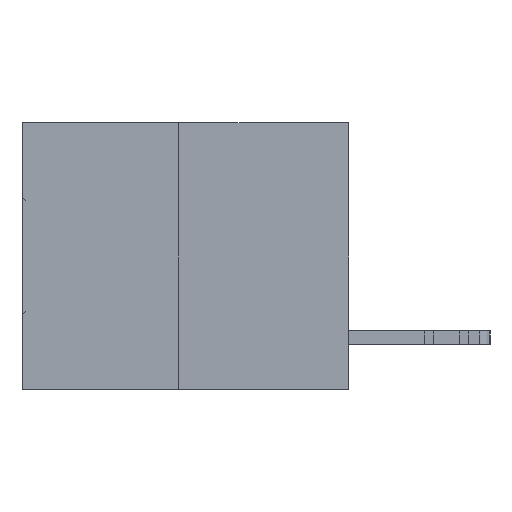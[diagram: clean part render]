
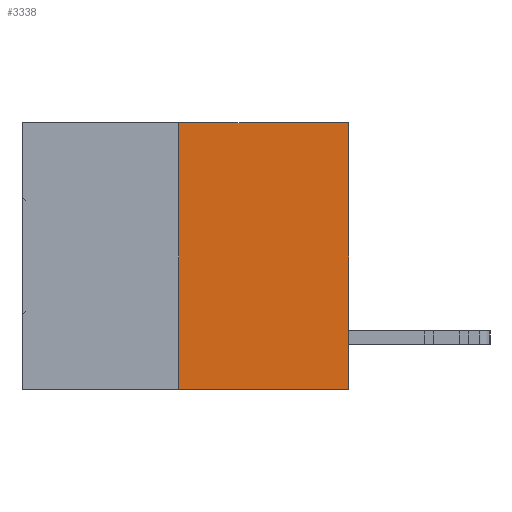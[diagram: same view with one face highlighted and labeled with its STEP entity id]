
A CAD part, left-side view. The second image highlights one B-rep face of the part: STEP entity #3338.
In plain terms, the highlighted planar face has unit normal (-1, 0, 0).
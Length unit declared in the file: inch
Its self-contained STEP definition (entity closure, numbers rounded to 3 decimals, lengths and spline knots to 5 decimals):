
#1250 = LINE ( 'NONE', #34219, #11824 ) ;
#2017 = CARTESIAN_POINT ( 'NONE',  ( 0., 0.312, -0.49 ) ) ;
#2782 = DIRECTION ( 'NONE',  ( 0., 0., -1. ) ) ;
#3338 = ADVANCED_FACE ( 'NONE', ( #34687 ), #34690, .F. ) ;
#3886 = CARTESIAN_POINT ( 'NONE',  ( 0., 0.6, -0.49 ) ) ;
#4591 = CARTESIAN_POINT ( 'NONE',  ( 0., 0.6, 0. ) ) ;
#6217 = CARTESIAN_POINT ( 'NONE',  ( 0., 0., 0. ) ) ;
#6683 = ORIENTED_EDGE ( 'NONE', *, *, #7709, .T. ) ;
#6906 = LINE ( 'NONE', #4591, #19614 ) ;
#7454 = VERTEX_POINT ( 'NONE', #23210 ) ;
#7709 = EDGE_CURVE ( 'NONE', #11153, #13397, #33931, .T. ) ;
#8301 = ORIENTED_EDGE ( 'NONE', *, *, #9869, .T. ) ;
#8942 = DIRECTION ( 'NONE',  ( 0., 0., 1. ) ) ;
#9840 = CARTESIAN_POINT ( 'NONE',  ( 0., 0., 0. ) ) ;
#9869 = EDGE_CURVE ( 'NONE', #22970, #11153, #18187, .T. ) ;
#10745 = DIRECTION ( 'NONE',  ( 1., 0., 0. ) ) ;
#10983 = VECTOR ( 'NONE', #31055, 39.37008 ) ;
#11153 = VERTEX_POINT ( 'NONE', #22570 ) ;
#11824 = VECTOR ( 'NONE', #8942, 39.37008 ) ;
#13397 = VERTEX_POINT ( 'NONE', #9840 ) ;
#13436 = EDGE_LOOP ( 'NONE', ( #29531, #8301, #6683, #24338 ) ) ;
#14988 = AXIS2_PLACEMENT_3D ( 'NONE', #32082, #10745, #2782 ) ;
#18187 = LINE ( 'NONE', #3886, #10983 ) ;
#19614 = VECTOR ( 'NONE', #25961, 39.37008 ) ;
#22570 = CARTESIAN_POINT ( 'NONE',  ( 0., 0., -0.49 ) ) ;
#22970 = VERTEX_POINT ( 'NONE', #2017 ) ;
#23210 = CARTESIAN_POINT ( 'NONE',  ( 0., 0.312, 0. ) ) ;
#24338 = ORIENTED_EDGE ( 'NONE', *, *, #32010, .F. ) ;
#25081 = DIRECTION ( 'NONE',  ( 0., 0., 1. ) ) ;
#25961 = DIRECTION ( 'NONE',  ( 0., -1., 0. ) ) ;
#26695 = VECTOR ( 'NONE', #25081, 39.37008 ) ;
#28719 = EDGE_CURVE ( 'NONE', #22970, #7454, #1250, .T. ) ;
#29531 = ORIENTED_EDGE ( 'NONE', *, *, #28719, .F. ) ;
#31055 = DIRECTION ( 'NONE',  ( 0., -1., 0. ) ) ;
#32010 = EDGE_CURVE ( 'NONE', #7454, #13397, #6906, .T. ) ;
#32082 = CARTESIAN_POINT ( 'NONE',  ( 0., 0.6, 0. ) ) ;
#33931 = LINE ( 'NONE', #6217, #26695 ) ;
#34219 = CARTESIAN_POINT ( 'NONE',  ( 0., 0.312, -0.49 ) ) ;
#34687 = FACE_OUTER_BOUND ( 'NONE', #13436, .T. ) ;
#34690 = PLANE ( 'NONE',  #14988 ) ;
